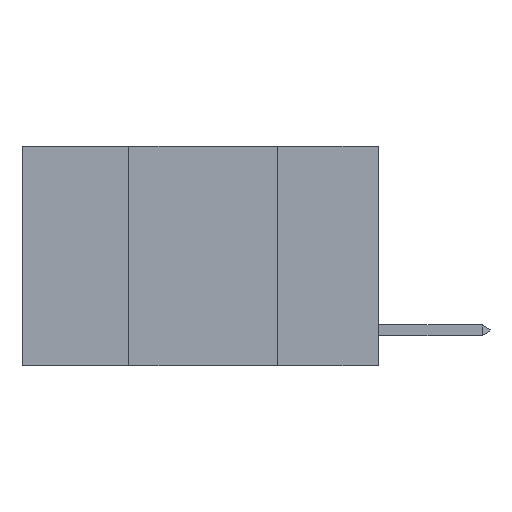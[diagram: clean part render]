
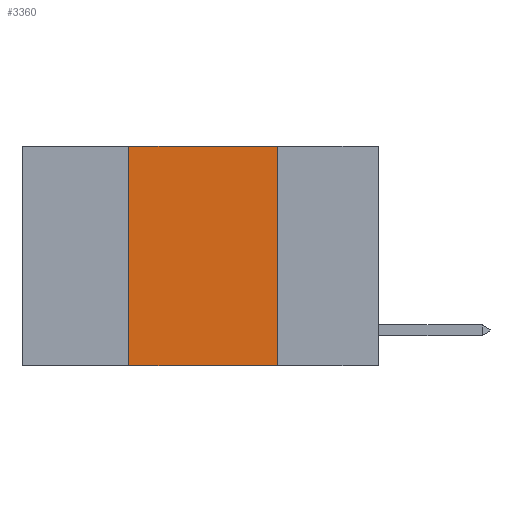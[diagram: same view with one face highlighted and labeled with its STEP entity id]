
A CAD part, left-side view. The second image highlights one B-rep face of the part: STEP entity #3360.
In plain terms, the highlighted planar face has unit normal (-1, 0, 0).
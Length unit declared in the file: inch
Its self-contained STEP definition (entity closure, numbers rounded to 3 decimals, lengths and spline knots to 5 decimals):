
#197 = CARTESIAN_POINT ( 'NONE',  ( 0., 0.17, 0. ) ) ;
#692 = CARTESIAN_POINT ( 'NONE',  ( 0., 0.42, 0. ) ) ;
#1215 = LINE ( 'NONE', #692, #12882 ) ;
#1222 = VECTOR ( 'NONE', #3233, 39.37008 ) ;
#1759 = DIRECTION ( 'NONE',  ( 1., 0., 0. ) ) ;
#1775 = VERTEX_POINT ( 'NONE', #16679 ) ;
#2937 = DIRECTION ( 'NONE',  ( 0., -1., 0. ) ) ;
#3233 = DIRECTION ( 'NONE',  ( 0., 0., -1. ) ) ;
#3238 = VERTEX_POINT ( 'NONE', #12064 ) ;
#3360 = ADVANCED_FACE ( 'NONE', ( #11772 ), #16976, .F. ) ;
#4590 = VECTOR ( 'NONE', #17847, 39.37008 ) ;
#5274 = LINE ( 'NONE', #197, #1222 ) ;
#5842 = LINE ( 'NONE', #15123, #14404 ) ;
#6673 = ORIENTED_EDGE ( 'NONE', *, *, #10836, .T. ) ;
#7586 = VERTEX_POINT ( 'NONE', #17494 ) ;
#8680 = CARTESIAN_POINT ( 'NONE',  ( 0., 0.6, -0.37 ) ) ;
#9583 = VERTEX_POINT ( 'NONE', #11847 ) ;
#9697 = EDGE_CURVE ( 'NONE', #7586, #3238, #5842, .T. ) ;
#10836 = EDGE_CURVE ( 'NONE', #9583, #1775, #12197, .T. ) ;
#11772 = FACE_OUTER_BOUND ( 'NONE', #19419, .T. ) ;
#11847 = CARTESIAN_POINT ( 'NONE',  ( 0., 0.42, -0.37 ) ) ;
#11865 = EDGE_CURVE ( 'NONE', #9583, #7586, #1215, .T. ) ;
#12064 = CARTESIAN_POINT ( 'NONE',  ( 0., 0.17, 0. ) ) ;
#12197 = LINE ( 'NONE', #8680, #4590 ) ;
#12286 = ORIENTED_EDGE ( 'NONE', *, *, #11865, .F. ) ;
#12397 = DIRECTION ( 'NONE',  ( 0., 0., -1. ) ) ;
#12678 = AXIS2_PLACEMENT_3D ( 'NONE', #15414, #1759, #12397 ) ;
#12869 = DIRECTION ( 'NONE',  ( 0., 0., 1. ) ) ;
#12882 = VECTOR ( 'NONE', #12869, 39.37008 ) ;
#12892 = EDGE_CURVE ( 'NONE', #3238, #1775, #5274, .T. ) ;
#14404 = VECTOR ( 'NONE', #2937, 39.37008 ) ;
#14643 = ORIENTED_EDGE ( 'NONE', *, *, #9697, .F. ) ;
#15123 = CARTESIAN_POINT ( 'NONE',  ( 0., 0.6, 0. ) ) ;
#15414 = CARTESIAN_POINT ( 'NONE',  ( 0., 0.6, 0. ) ) ;
#16679 = CARTESIAN_POINT ( 'NONE',  ( 0., 0.17, -0.37 ) ) ;
#16976 = PLANE ( 'NONE',  #12678 ) ;
#17494 = CARTESIAN_POINT ( 'NONE',  ( 0., 0.42, 0. ) ) ;
#17847 = DIRECTION ( 'NONE',  ( 0., -1., 0. ) ) ;
#19021 = ORIENTED_EDGE ( 'NONE', *, *, #12892, .F. ) ;
#19419 = EDGE_LOOP ( 'NONE', ( #19021, #14643, #12286, #6673 ) ) ;
